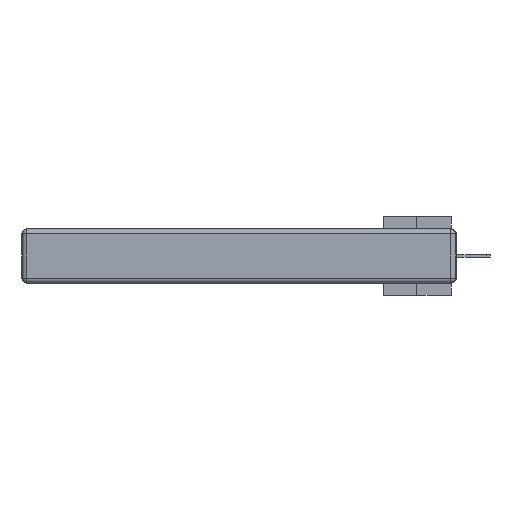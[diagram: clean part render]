
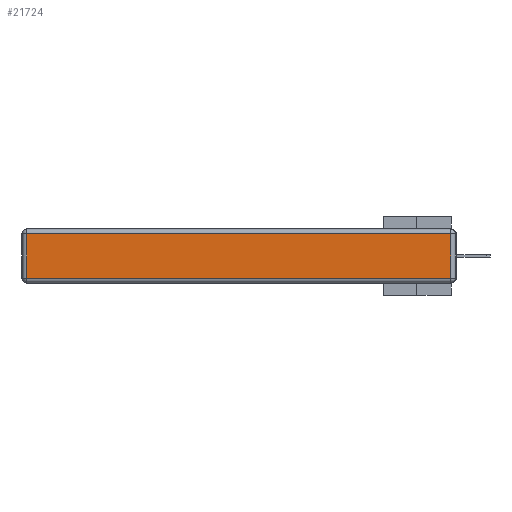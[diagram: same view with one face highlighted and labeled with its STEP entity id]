
A CAD part, left-side view. The second image highlights one B-rep face of the part: STEP entity #21724.
In plain terms, the highlighted planar face has unit normal (-1, 0, 0).
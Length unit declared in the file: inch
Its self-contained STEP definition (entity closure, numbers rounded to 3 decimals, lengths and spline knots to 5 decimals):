
#393 = EDGE_CURVE ( 'NONE', #2260, #1447, #24241, .T. ) ;
#477 = PLANE ( 'NONE',  #11237 ) ;
#1275 = VECTOR ( 'NONE', #13371, 39.37008 ) ;
#1447 = VERTEX_POINT ( 'NONE', #30341 ) ;
#1740 = VECTOR ( 'NONE', #35188, 39.37008 ) ;
#2260 = VERTEX_POINT ( 'NONE', #22734 ) ;
#2687 = LINE ( 'NONE', #14472, #1740 ) ;
#3131 = EDGE_LOOP ( 'NONE', ( #9604, #26494, #31363, #9150 ) ) ;
#3507 = DIRECTION ( 'NONE',  ( 0., 0., 1. ) ) ;
#6495 = DIRECTION ( 'NONE',  ( -1., 0., 0. ) ) ;
#9150 = ORIENTED_EDGE ( 'NONE', *, *, #33345, .T. ) ;
#9604 = ORIENTED_EDGE ( 'NONE', *, *, #32445, .T. ) ;
#10867 = CARTESIAN_POINT ( 'NONE',  ( 0., 2.72, -0.03 ) ) ;
#11237 = AXIS2_PLACEMENT_3D ( 'NONE', #36300, #6495, #3507 ) ;
#11390 = VECTOR ( 'NONE', #16276, 39.37008 ) ;
#13371 = DIRECTION ( 'NONE',  ( 0., -1., 0. ) ) ;
#14472 = CARTESIAN_POINT ( 'NONE',  ( 0., 2.72, -0.343 ) ) ;
#15990 = VERTEX_POINT ( 'NONE', #27178 ) ;
#16276 = DIRECTION ( 'NONE',  ( 0., 1., 0. ) ) ;
#18332 = LINE ( 'NONE', #19333, #1275 ) ;
#18549 = VERTEX_POINT ( 'NONE', #10867 ) ;
#19333 = CARTESIAN_POINT ( 'NONE',  ( 0., 0., -0.313 ) ) ;
#21724 = ADVANCED_FACE ( 'NONE', ( #22090 ), #477, .T. ) ;
#22090 = FACE_OUTER_BOUND ( 'NONE', #3131, .T. ) ;
#22605 = EDGE_CURVE ( 'NONE', #1447, #18549, #35951, .T. ) ;
#22734 = CARTESIAN_POINT ( 'NONE',  ( 0., 0.03, -0.313 ) ) ;
#24241 = LINE ( 'NONE', #33852, #31213 ) ;
#26494 = ORIENTED_EDGE ( 'NONE', *, *, #393, .T. ) ;
#27178 = CARTESIAN_POINT ( 'NONE',  ( 0., 2.72, -0.313 ) ) ;
#30341 = CARTESIAN_POINT ( 'NONE',  ( 0., 0.03, -0.03 ) ) ;
#30986 = CARTESIAN_POINT ( 'NONE',  ( 0., 2.75, -0.03 ) ) ;
#31213 = VECTOR ( 'NONE', #33641, 39.37008 ) ;
#31363 = ORIENTED_EDGE ( 'NONE', *, *, #22605, .T. ) ;
#32445 = EDGE_CURVE ( 'NONE', #15990, #2260, #18332, .T. ) ;
#33345 = EDGE_CURVE ( 'NONE', #18549, #15990, #2687, .T. ) ;
#33641 = DIRECTION ( 'NONE',  ( 0., 0., 1. ) ) ;
#33852 = CARTESIAN_POINT ( 'NONE',  ( 0., 0.03, -0.343 ) ) ;
#35188 = DIRECTION ( 'NONE',  ( 0., 0., -1. ) ) ;
#35951 = LINE ( 'NONE', #30986, #11390 ) ;
#36300 = CARTESIAN_POINT ( 'NONE',  ( 0., 0., -0.343 ) ) ;
